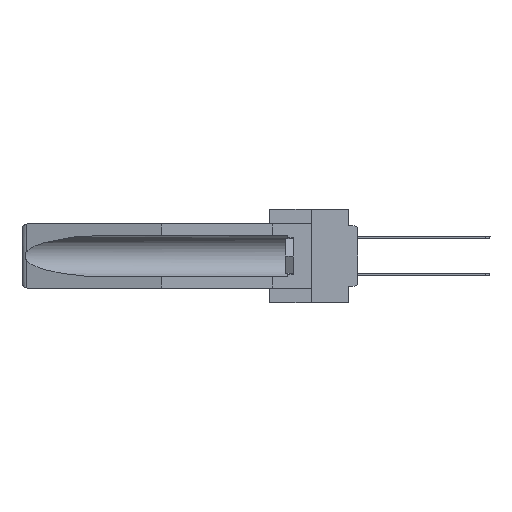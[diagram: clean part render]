
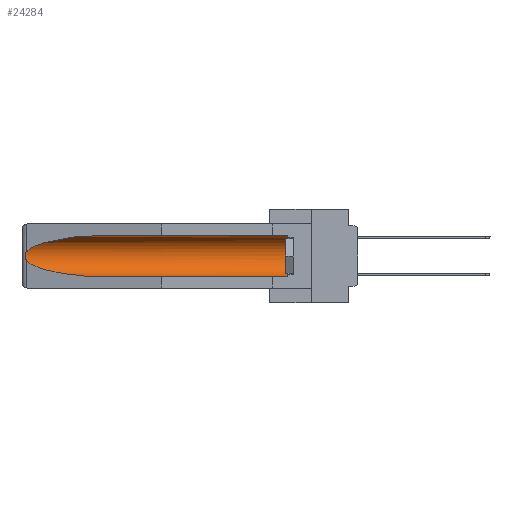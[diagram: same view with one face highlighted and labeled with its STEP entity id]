
A CAD part, left-side view. The second image highlights one B-rep face of the part: STEP entity #24284.
In plain terms, the highlighted cylindrical face has radius 2.857 mm (diameter 5.715 mm), a partial arc.
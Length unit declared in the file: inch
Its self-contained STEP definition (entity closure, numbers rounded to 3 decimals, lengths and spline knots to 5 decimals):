
#213 = CARTESIAN_POINT ( 'NONE',  ( 0.155, -0.30754, -0.284 ) ) ;
#390 = AXIS2_PLACEMENT_3D ( 'NONE', #12850, #22087, #17511 ) ;
#571 = CARTESIAN_POINT ( 'NONE',  ( 0.26537, 1.52718, -0.19328 ) ) ;
#2794 = CARTESIAN_POINT ( 'NONE',  ( 0.26537, 1.52718, -0.14972 ) ) ;
#2823 = CARTESIAN_POINT ( 'NONE',  ( 0.2673, 1.53269, -0.17917 ) ) ;
#2981 = CARTESIAN_POINT ( 'NONE',  ( 0.2673, 1.5327, -0.16383 ) ) ;
#3029 = VECTOR ( 'NONE', #10956, 39.37008 ) ;
#3103 = CARTESIAN_POINT ( 'NONE',  ( 0.26537, 1.52718, -0.14972 ) ) ;
#3719 = CARTESIAN_POINT ( 'NONE',  ( 0.25451, 1.48313, -0.24835 ) ) ;
#5148 = CARTESIAN_POINT ( 'NONE',  ( 0.26655, 1.53094, -0.18657 ) ) ;
#5640 = VERTEX_POINT ( 'NONE', #3103 ) ;
#5868 = ORIENTED_EDGE ( 'NONE', *, *, #9711, .F. ) ;
#5913 = EDGE_CURVE ( 'NONE', #17834, #14346, #18555, .T. ) ;
#6048 = EDGE_LOOP ( 'NONE', ( #16734, #8111, #18211, #5868, #17681, #9368 ) ) ;
#6321 = CARTESIAN_POINT ( 'NONE',  ( 0.155, 1.07973, -0.284 ) ) ;
#6519 = DIRECTION ( 'NONE',  ( 0., 0., 1. ) ) ;
#6726 = CARTESIAN_POINT ( 'NONE',  ( 0.155, 0.126, -0.284 ) ) ;
#6930 = AXIS2_PLACEMENT_3D ( 'NONE', #8862, #22248, #6519 ) ;
#7659 = VECTOR ( 'NONE', #24641, 39.37008 ) ;
#7919 = EDGE_CURVE ( 'NONE', #15680, #17834, #28245, .T. ) ;
#8111 = ORIENTED_EDGE ( 'NONE', *, *, #18313, .T. ) ;
#8862 = CARTESIAN_POINT ( 'NONE',  ( 0.155, -0.30754, -0.1715 ) ) ;
#9368 = ORIENTED_EDGE ( 'NONE', *, *, #5913, .T. ) ;
#9654 = CARTESIAN_POINT ( 'NONE',  ( 0.21114, 1.30732, -0.059 ) ) ;
#9711 = EDGE_CURVE ( 'NONE', #15680, #18935, #20320, .T. ) ;
#10240 = VERTEX_POINT ( 'NONE', #571 ) ;
#10956 = DIRECTION ( 'NONE',  ( 0., 1., 0. ) ) ;
#11751 = CARTESIAN_POINT ( 'NONE',  ( 0.2675, 1.53308, -0.17534 ) ) ;
#11876 = CARTESIAN_POINT ( 'NONE',  ( 0.25451, 1.48313, -0.09465 ) ) ;
#12850 = CARTESIAN_POINT ( 'NONE',  ( 0.155, 0.126, -0.1715 ) ) ;
#13946 = CARTESIAN_POINT ( 'NONE',  ( 0.2675, 1.53308, -0.16763 ) ) ;
#14346 = VERTEX_POINT ( 'NONE', #20501 ) ;
#14348 = CARTESIAN_POINT ( 'NONE',  ( 0.155, 1.07973, -0.059 ) ) ;
#14385 = CARTESIAN_POINT ( 'NONE',  ( 0.26597, 1.5296, -0.19026 ) ) ;
#15680 = VERTEX_POINT ( 'NONE', #6726 ) ;
#16450 = CARTESIAN_POINT ( 'NONE',  ( 0.26537, 1.52718, -0.14972 ) ) ;
#16595 = CARTESIAN_POINT ( 'NONE',  ( 0.26597, 1.52961, -0.15275 ) ) ;
#16734 = ORIENTED_EDGE ( 'NONE', *, *, #20071, .T. ) ;
#16744 = CARTESIAN_POINT ( 'NONE',  ( 0.26537, 1.52718, -0.19328 ) ) ;
#17511 = DIRECTION ( 'NONE',  ( 0., 0., 1. ) ) ;
#17651 = FACE_OUTER_BOUND ( 'NONE', #6048, .T. ) ;
#17681 = ORIENTED_EDGE ( 'NONE', *, *, #7919, .T. ) ;
#17834 = VERTEX_POINT ( 'NONE', #24587 ) ;
#18164 = B_SPLINE_CURVE_WITH_KNOTS ( 'NONE', 3,
 ( #16450, #16595, #20846, #2981, #13946, #11751, #2823, #5148, #14385, #16744 ),
 .UNSPECIFIED., .F., .F.,
 ( 4, 2, 2, 2, 4 ),
 ( 0., 0.00029, 0.00058, 0.00087, 0.00117 ),
 .UNSPECIFIED. ) ;
#18211 = ORIENTED_EDGE ( 'NONE', *, *, #19778, .T. ) ;
#18313 = EDGE_CURVE ( 'NONE', #5640, #10240, #18164, .T. ) ;
#18555 = LINE ( 'NONE', #27295, #7659 ) ;
#18935 = VERTEX_POINT ( 'NONE', #28059 ) ;
#19518 = CARTESIAN_POINT ( 'NONE',  ( 0.21114, 1.30732, -0.284 ) ) ;
#19778 = EDGE_CURVE ( 'NONE', #10240, #18935, #26197, .T. ) ;
#20071 = EDGE_CURVE ( 'NONE', #14346, #5640, #24121, .T. ) ;
#20150 = CYLINDRICAL_SURFACE ( 'NONE', #6930, 0.1125 ) ;
#20320 = LINE ( 'NONE', #213, #3029 ) ;
#20501 = CARTESIAN_POINT ( 'NONE',  ( 0.155, 1.07973, -0.059 ) ) ;
#20846 = CARTESIAN_POINT ( 'NONE',  ( 0.26654, 1.53092, -0.15636 ) ) ;
#21465 = CARTESIAN_POINT ( 'NONE',  ( 0.26537, 1.52718, -0.19328 ) ) ;
#22087 = DIRECTION ( 'NONE',  ( 0., -1., 0. ) ) ;
#22248 = DIRECTION ( 'NONE',  ( 0., 1., 0. ) ) ;
#24121 =( BOUNDED_CURVE ( )  B_SPLINE_CURVE ( 3, ( #14348, #9654, #11876, #2794 ),
 .UNSPECIFIED., .F., .T. ) 
 B_SPLINE_CURVE_WITH_KNOTS ( ( 4, 4 ),
 ( 4.71239, 6.08839 ),
 .UNSPECIFIED. ) 
 CURVE ( )  GEOMETRIC_REPRESENTATION_ITEM ( )  RATIONAL_B_SPLINE_CURVE ( ( 1., 0.848, 0.848, 1. ) ) 
 REPRESENTATION_ITEM ( '' )  );
#24284 = ADVANCED_FACE ( 'NONE', ( #17651 ), #20150, .F. ) ;
#24587 = CARTESIAN_POINT ( 'NONE',  ( 0.155, 0.126, -0.059 ) ) ;
#24641 = DIRECTION ( 'NONE',  ( 0., 1., 0. ) ) ;
#26197 =( BOUNDED_CURVE ( )  B_SPLINE_CURVE ( 3, ( #21465, #3719, #19518, #6321 ),
 .UNSPECIFIED., .F., .T. ) 
 B_SPLINE_CURVE_WITH_KNOTS ( ( 4, 4 ),
 ( 0.1948, 1.5708 ),
 .UNSPECIFIED. ) 
 CURVE ( )  GEOMETRIC_REPRESENTATION_ITEM ( )  RATIONAL_B_SPLINE_CURVE ( ( 1., 0.848, 0.848, 1. ) ) 
 REPRESENTATION_ITEM ( '' )  );
#27295 = CARTESIAN_POINT ( 'NONE',  ( 0.155, -0.30754, -0.059 ) ) ;
#28059 = CARTESIAN_POINT ( 'NONE',  ( 0.155, 1.07973, -0.284 ) ) ;
#28245 = CIRCLE ( 'NONE', #390, 0.1125 ) ;
